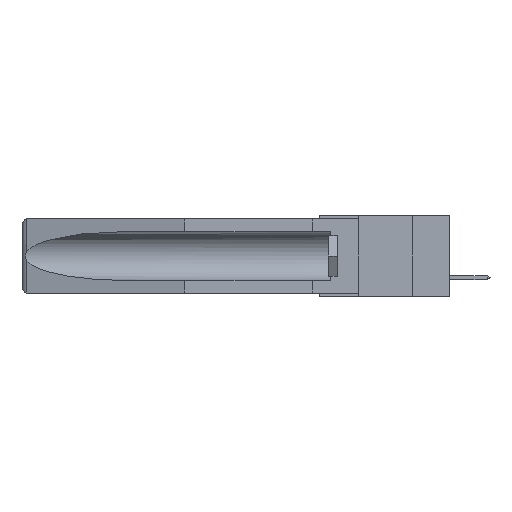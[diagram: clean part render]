
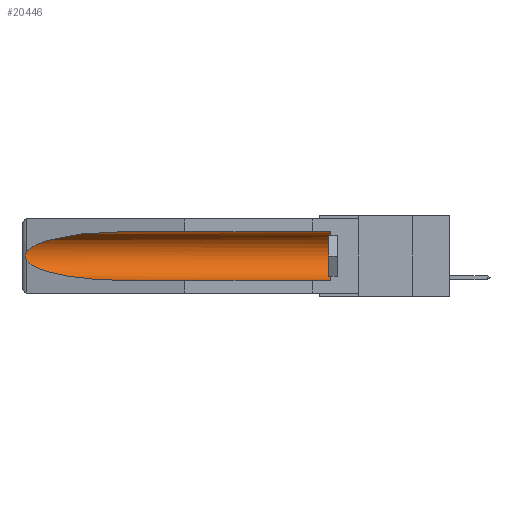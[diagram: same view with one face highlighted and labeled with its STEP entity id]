
A CAD part, left-side view. The second image highlights one B-rep face of the part: STEP entity #20446.
In plain terms, the highlighted cylindrical face has radius 2.857 mm (diameter 5.715 mm), a partial arc.
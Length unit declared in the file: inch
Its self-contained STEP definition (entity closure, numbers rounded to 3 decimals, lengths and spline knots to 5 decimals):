
#24 = EDGE_CURVE ( 'NONE', #30308, #29756, #10758, .T. ) ;
#160 = CARTESIAN_POINT ( 'NONE',  ( 0.155, -0.30754, -0.284 ) ) ;
#266 = DIRECTION ( 'NONE',  ( 0., 1., 0. ) ) ;
#1812 = CARTESIAN_POINT ( 'NONE',  ( 0.2675, 1.53308, -0.16763 ) ) ;
#2015 = CARTESIAN_POINT ( 'NONE',  ( 0.26654, 1.53092, -0.15636 ) ) ;
#3480 = CARTESIAN_POINT ( 'NONE',  ( 0.155, 1.07973, -0.284 ) ) ;
#4435 = CARTESIAN_POINT ( 'NONE',  ( 0.2673, 1.5327, -0.16383 ) ) ;
#4720 = ORIENTED_EDGE ( 'NONE', *, *, #9045, .T. ) ;
#4729 = VECTOR ( 'NONE', #266, 39.37008 ) ;
#4856 = CARTESIAN_POINT ( 'NONE',  ( 0.155, 1.07973, -0.284 ) ) ;
#5097 = EDGE_LOOP ( 'NONE', ( #14632, #6918, #4720, #14986, #7431, #14529 ) ) ;
#5767 = VERTEX_POINT ( 'NONE', #9451 ) ;
#5968 = VERTEX_POINT ( 'NONE', #4856 ) ;
#6729 = CARTESIAN_POINT ( 'NONE',  ( 0.2675, 1.53308, -0.17534 ) ) ;
#6825 = CARTESIAN_POINT ( 'NONE',  ( 0.25451, 1.48313, -0.09465 ) ) ;
#6904 = CARTESIAN_POINT ( 'NONE',  ( 0.26537, 1.52718, -0.14972 ) ) ;
#6918 = ORIENTED_EDGE ( 'NONE', *, *, #26467, .T. ) ;
#7431 = ORIENTED_EDGE ( 'NONE', *, *, #24, .T. ) ;
#7611 =( BOUNDED_CURVE ( )  B_SPLINE_CURVE ( 3, ( #17758, #22521, #27552, #3480 ),
 .UNSPECIFIED., .F., .F. ) 
 B_SPLINE_CURVE_WITH_KNOTS ( ( 4, 4 ),
 ( 0.1948, 1.5708 ),
 .UNSPECIFIED. ) 
 CURVE ( )  GEOMETRIC_REPRESENTATION_ITEM ( )  RATIONAL_B_SPLINE_CURVE ( ( 1., 0.848, 0.848, 1. ) ) 
 REPRESENTATION_ITEM ( '' )  );
#7976 =( BOUNDED_CURVE ( )  B_SPLINE_CURVE ( 3, ( #11321, #16107, #6825, #13723 ),
 .UNSPECIFIED., .F., .F. ) 
 B_SPLINE_CURVE_WITH_KNOTS ( ( 4, 4 ),
 ( 4.71239, 6.08839 ),
 .UNSPECIFIED. ) 
 CURVE ( )  GEOMETRIC_REPRESENTATION_ITEM ( )  RATIONAL_B_SPLINE_CURVE ( ( 1., 0.848, 0.848, 1. ) ) 
 REPRESENTATION_ITEM ( '' )  );
#8855 = EDGE_CURVE ( 'NONE', #29756, #5767, #13992, .T. ) ;
#9045 = EDGE_CURVE ( 'NONE', #11821, #5968, #7611, .T. ) ;
#9451 = CARTESIAN_POINT ( 'NONE',  ( 0.155, 1.07973, -0.059 ) ) ;
#9889 = VECTOR ( 'NONE', #29224, 39.37008 ) ;
#10087 = DIRECTION ( 'NONE',  ( 0., -1., 0. ) ) ;
#10675 = AXIS2_PLACEMENT_3D ( 'NONE', #17379, #10087, #26726 ) ;
#10758 = CIRCLE ( 'NONE', #10675, 0.1125 ) ;
#11321 = CARTESIAN_POINT ( 'NONE',  ( 0.155, 1.07973, -0.059 ) ) ;
#11455 = DIRECTION ( 'NONE',  ( 0., 1., 0. ) ) ;
#11821 = VERTEX_POINT ( 'NONE', #27964 ) ;
#12617 = CARTESIAN_POINT ( 'NONE',  ( 0.155, -0.30754, -0.059 ) ) ;
#13723 = CARTESIAN_POINT ( 'NONE',  ( 0.26537, 1.52718, -0.14972 ) ) ;
#13732 = CARTESIAN_POINT ( 'NONE',  ( 0.26655, 1.53094, -0.18657 ) ) ;
#13992 = LINE ( 'NONE', #12617, #9889 ) ;
#14529 = ORIENTED_EDGE ( 'NONE', *, *, #8855, .T. ) ;
#14632 = ORIENTED_EDGE ( 'NONE', *, *, #15010, .T. ) ;
#14814 = FACE_OUTER_BOUND ( 'NONE', #5097, .T. ) ;
#14986 = ORIENTED_EDGE ( 'NONE', *, *, #20546, .F. ) ;
#15010 = EDGE_CURVE ( 'NONE', #5767, #30549, #7976, .T. ) ;
#16107 = CARTESIAN_POINT ( 'NONE',  ( 0.21114, 1.30732, -0.059 ) ) ;
#16443 = DIRECTION ( 'NONE',  ( 0., 0., 1. ) ) ;
#17379 = CARTESIAN_POINT ( 'NONE',  ( 0.155, 0.126, -0.1715 ) ) ;
#17403 = LINE ( 'NONE', #160, #4729 ) ;
#17758 = CARTESIAN_POINT ( 'NONE',  ( 0.26537, 1.52718, -0.19328 ) ) ;
#18795 = CARTESIAN_POINT ( 'NONE',  ( 0.2673, 1.53269, -0.17917 ) ) ;
#19283 = CARTESIAN_POINT ( 'NONE',  ( 0.155, 0.126, -0.059 ) ) ;
#19984 = CYLINDRICAL_SURFACE ( 'NONE', #25694, 0.1125 ) ;
#20446 = ADVANCED_FACE ( 'NONE', ( #14814 ), #19984, .F. ) ;
#20546 = EDGE_CURVE ( 'NONE', #30308, #5968, #17403, .T. ) ;
#21080 = CARTESIAN_POINT ( 'NONE',  ( 0.26537, 1.52718, -0.19328 ) ) ;
#22521 = CARTESIAN_POINT ( 'NONE',  ( 0.25451, 1.48313, -0.24835 ) ) ;
#23260 = CARTESIAN_POINT ( 'NONE',  ( 0.26537, 1.52718, -0.14972 ) ) ;
#23367 = CARTESIAN_POINT ( 'NONE',  ( 0.26597, 1.5296, -0.19026 ) ) ;
#25665 = CARTESIAN_POINT ( 'NONE',  ( 0.26597, 1.52961, -0.15275 ) ) ;
#25694 = AXIS2_PLACEMENT_3D ( 'NONE', #28168, #11455, #16443 ) ;
#26467 = EDGE_CURVE ( 'NONE', #30549, #11821, #29719, .T. ) ;
#26726 = DIRECTION ( 'NONE',  ( 0., 0., 1. ) ) ;
#27552 = CARTESIAN_POINT ( 'NONE',  ( 0.21114, 1.30732, -0.284 ) ) ;
#27964 = CARTESIAN_POINT ( 'NONE',  ( 0.26537, 1.52718, -0.19328 ) ) ;
#28168 = CARTESIAN_POINT ( 'NONE',  ( 0.155, -0.30754, -0.1715 ) ) ;
#29224 = DIRECTION ( 'NONE',  ( 0., 1., 0. ) ) ;
#29460 = CARTESIAN_POINT ( 'NONE',  ( 0.155, 0.126, -0.284 ) ) ;
#29719 = B_SPLINE_CURVE_WITH_KNOTS ( 'NONE', 3,
 ( #23260, #25665, #2015, #4435, #1812, #6729, #18795, #13732, #23367, #21080 ),
 .UNSPECIFIED., .F., .F.,
 ( 4, 2, 2, 2, 4 ),
 ( 0., 0.00029, 0.00058, 0.00087, 0.00117 ),
 .UNSPECIFIED. ) ;
#29756 = VERTEX_POINT ( 'NONE', #19283 ) ;
#30308 = VERTEX_POINT ( 'NONE', #29460 ) ;
#30549 = VERTEX_POINT ( 'NONE', #6904 ) ;
